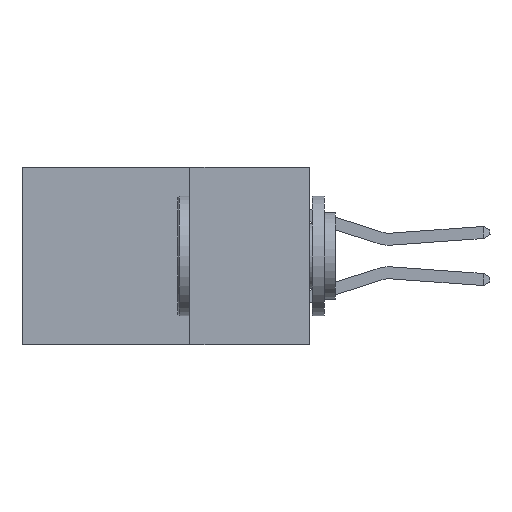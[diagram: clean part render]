
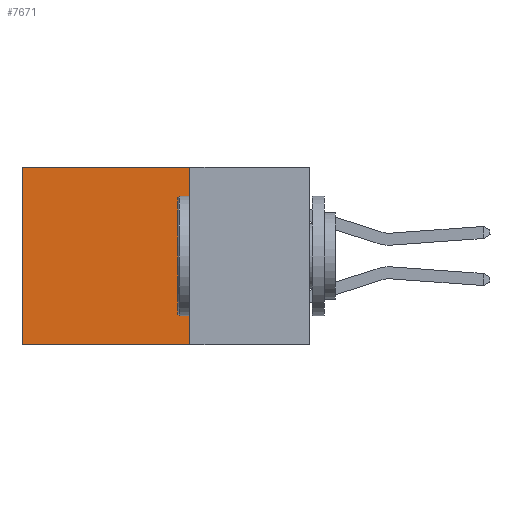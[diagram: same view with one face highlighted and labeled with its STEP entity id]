
A CAD part, left-side view. The second image highlights one B-rep face of the part: STEP entity #7671.
In plain terms, the highlighted planar face has unit normal (-1, 0, 0).
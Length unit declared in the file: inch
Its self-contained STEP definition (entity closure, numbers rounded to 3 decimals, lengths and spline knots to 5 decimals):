
#503 = PLANE ( 'NONE',  #5362 ) ;
#683 = CARTESIAN_POINT ( 'NONE',  ( 0.2615, 0.6, 0. ) ) ;
#689 = DIRECTION ( 'NONE',  ( 0., 0., -1. ) ) ;
#726 = DIRECTION ( 'NONE',  ( 0., 0., -1. ) ) ;
#817 = DIRECTION ( 'NONE',  ( 0., 1., 0. ) ) ;
#979 = EDGE_CURVE ( 'NONE', #8837, #3657, #4281, .T. ) ;
#987 = ORIENTED_EDGE ( 'NONE', *, *, #4091, .F. ) ;
#1173 = LINE ( 'NONE', #9602, #8842 ) ;
#2176 = CARTESIAN_POINT ( 'NONE',  ( 0.2615, 0.6, -0.37 ) ) ;
#2598 = EDGE_CURVE ( 'NONE', #9509, #8261, #5247, .T. ) ;
#2671 = EDGE_LOOP ( 'NONE', ( #4743, #987, #3236, #2954 ) ) ;
#2954 = ORIENTED_EDGE ( 'NONE', *, *, #2976, .T. ) ;
#2976 = EDGE_CURVE ( 'NONE', #8837, #9509, #9157, .T. ) ;
#3236 = ORIENTED_EDGE ( 'NONE', *, *, #979, .F. ) ;
#3657 = VERTEX_POINT ( 'NONE', #8044 ) ;
#4091 = EDGE_CURVE ( 'NONE', #3657, #8261, #1173, .T. ) ;
#4132 = CARTESIAN_POINT ( 'NONE',  ( 0.2615, 0.25, 0. ) ) ;
#4281 = LINE ( 'NONE', #4420, #5262 ) ;
#4282 = DIRECTION ( 'NONE',  ( 1., 0., 0. ) ) ;
#4420 = CARTESIAN_POINT ( 'NONE',  ( 0.2615, 0.25, -0.37 ) ) ;
#4743 = ORIENTED_EDGE ( 'NONE', *, *, #2598, .T. ) ;
#5247 = LINE ( 'NONE', #2176, #9055 ) ;
#5262 = VECTOR ( 'NONE', #6543, 39.37008 ) ;
#5362 = AXIS2_PLACEMENT_3D ( 'NONE', #6634, #4282, #689 ) ;
#6122 = CARTESIAN_POINT ( 'NONE',  ( 0.2615, 0.25, 0. ) ) ;
#6543 = DIRECTION ( 'NONE',  ( 0., 0., -1. ) ) ;
#6634 = CARTESIAN_POINT ( 'NONE',  ( 0.2615, 0.25, -0.37 ) ) ;
#7671 = ADVANCED_FACE ( 'NONE', ( #8224 ), #503, .F. ) ;
#7832 = VECTOR ( 'NONE', #817, 39.37008 ) ;
#8044 = CARTESIAN_POINT ( 'NONE',  ( 0.2615, 0.25, -0.37 ) ) ;
#8072 = DIRECTION ( 'NONE',  ( 0., 1., 0. ) ) ;
#8224 = FACE_OUTER_BOUND ( 'NONE', #2671, .T. ) ;
#8261 = VERTEX_POINT ( 'NONE', #9072 ) ;
#8837 = VERTEX_POINT ( 'NONE', #4132 ) ;
#8842 = VECTOR ( 'NONE', #8072, 39.37008 ) ;
#9055 = VECTOR ( 'NONE', #726, 39.37008 ) ;
#9072 = CARTESIAN_POINT ( 'NONE',  ( 0.2615, 0.6, -0.37 ) ) ;
#9157 = LINE ( 'NONE', #6122, #7832 ) ;
#9509 = VERTEX_POINT ( 'NONE', #683 ) ;
#9602 = CARTESIAN_POINT ( 'NONE',  ( 0.2615, 0.25, -0.37 ) ) ;
